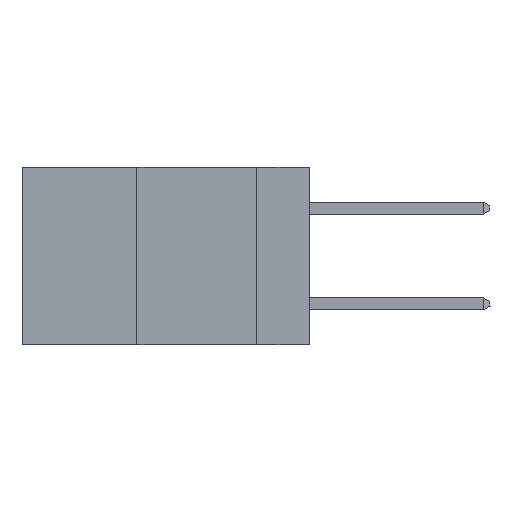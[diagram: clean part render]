
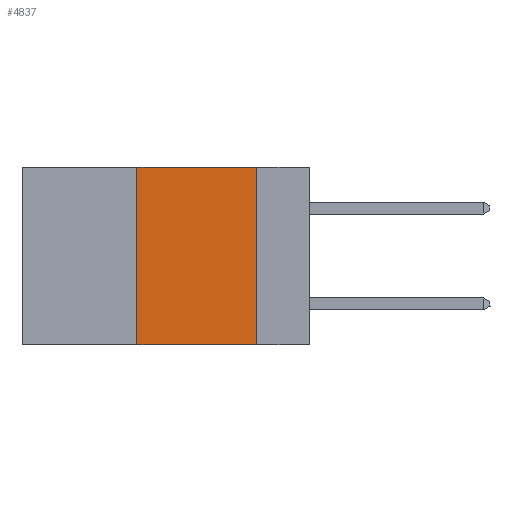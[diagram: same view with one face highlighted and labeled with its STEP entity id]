
A CAD part, left-side view. The second image highlights one B-rep face of the part: STEP entity #4837.
In plain terms, the highlighted planar face has unit normal (-1, 0, 0).
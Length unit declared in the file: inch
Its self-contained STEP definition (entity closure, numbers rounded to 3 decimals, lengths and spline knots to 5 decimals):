
#187 = EDGE_CURVE ( 'NONE', #8203, #3008, #4501, .T. ) ;
#268 = VECTOR ( 'NONE', #6227, 39.37008 ) ;
#296 = ORIENTED_EDGE ( 'NONE', *, *, #187, .F. ) ;
#377 = CARTESIAN_POINT ( 'NONE',  ( 0., 0.36, -0.37 ) ) ;
#1114 = CARTESIAN_POINT ( 'NONE',  ( 0., 0.6, 0. ) ) ;
#1187 = DIRECTION ( 'NONE',  ( 0., -1., 0. ) ) ;
#2106 = LINE ( 'NONE', #8315, #3600 ) ;
#2294 = CARTESIAN_POINT ( 'NONE',  ( 0., 0.11, -0.37 ) ) ;
#2395 = EDGE_LOOP ( 'NONE', ( #6582, #7472, #296, #6165 ) ) ;
#2887 = DIRECTION ( 'NONE',  ( 0., -1., 0. ) ) ;
#3008 = VERTEX_POINT ( 'NONE', #5137 ) ;
#3128 = LINE ( 'NONE', #8286, #7222 ) ;
#3143 = EDGE_CURVE ( 'NONE', #5456, #4558, #3128, .T. ) ;
#3600 = VECTOR ( 'NONE', #2887, 39.37008 ) ;
#3828 = FACE_OUTER_BOUND ( 'NONE', #2395, .T. ) ;
#3857 = EDGE_CURVE ( 'NONE', #8203, #4558, #2106, .T. ) ;
#4501 = LINE ( 'NONE', #8589, #268 ) ;
#4558 = VERTEX_POINT ( 'NONE', #2294 ) ;
#4592 = PLANE ( 'NONE',  #7543 ) ;
#4837 = ADVANCED_FACE ( 'NONE', ( #3828 ), #4592, .F. ) ;
#5137 = CARTESIAN_POINT ( 'NONE',  ( 0., 0.36, 0. ) ) ;
#5456 = VERTEX_POINT ( 'NONE', #6429 ) ;
#5469 = CARTESIAN_POINT ( 'NONE',  ( 0., 0.6, 0. ) ) ;
#6164 = DIRECTION ( 'NONE',  ( 1., 0., 0. ) ) ;
#6165 = ORIENTED_EDGE ( 'NONE', *, *, #3857, .T. ) ;
#6227 = DIRECTION ( 'NONE',  ( 0., 0., 1. ) ) ;
#6429 = CARTESIAN_POINT ( 'NONE',  ( 0., 0.11, 0. ) ) ;
#6462 = LINE ( 'NONE', #1114, #8541 ) ;
#6582 = ORIENTED_EDGE ( 'NONE', *, *, #3143, .F. ) ;
#7222 = VECTOR ( 'NONE', #7471, 39.37008 ) ;
#7471 = DIRECTION ( 'NONE',  ( 0., 0., -1. ) ) ;
#7472 = ORIENTED_EDGE ( 'NONE', *, *, #8516, .F. ) ;
#7543 = AXIS2_PLACEMENT_3D ( 'NONE', #5469, #6164, #10103 ) ;
#8203 = VERTEX_POINT ( 'NONE', #377 ) ;
#8286 = CARTESIAN_POINT ( 'NONE',  ( 0., 0.11, 0. ) ) ;
#8315 = CARTESIAN_POINT ( 'NONE',  ( 0., 0.6, -0.37 ) ) ;
#8516 = EDGE_CURVE ( 'NONE', #3008, #5456, #6462, .T. ) ;
#8541 = VECTOR ( 'NONE', #1187, 39.37008 ) ;
#8589 = CARTESIAN_POINT ( 'NONE',  ( 0., 0.36, 0. ) ) ;
#10103 = DIRECTION ( 'NONE',  ( 0., 0., -1. ) ) ;
